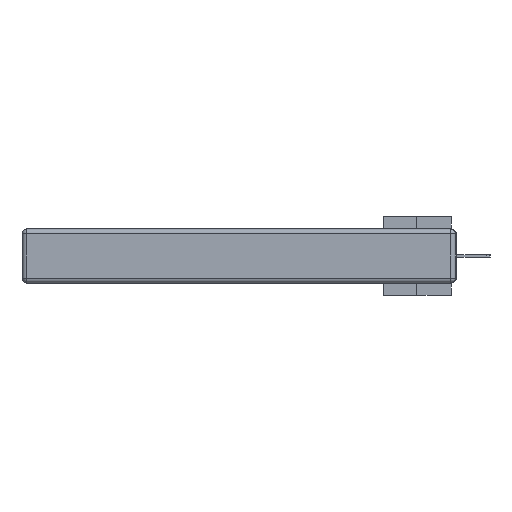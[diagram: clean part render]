
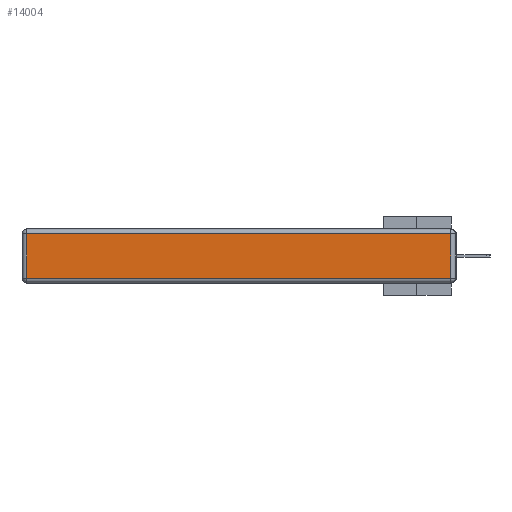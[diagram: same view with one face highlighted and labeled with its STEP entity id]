
A CAD part, left-side view. The second image highlights one B-rep face of the part: STEP entity #14004.
In plain terms, the highlighted planar face has unit normal (-1, 0, 0).
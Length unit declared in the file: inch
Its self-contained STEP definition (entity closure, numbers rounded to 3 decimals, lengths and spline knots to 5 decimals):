
#1077 = LINE ( 'NONE', #28165, #17261 ) ;
#1155 = ORIENTED_EDGE ( 'NONE', *, *, #31977, .T. ) ;
#1586 = CARTESIAN_POINT ( 'NONE',  ( 0., 0., -0.343 ) ) ;
#5888 = CARTESIAN_POINT ( 'NONE',  ( 0., 2.72, -0.313 ) ) ;
#6459 = VECTOR ( 'NONE', #10305, 39.37008 ) ;
#8306 = LINE ( 'NONE', #8474, #25198 ) ;
#8474 = CARTESIAN_POINT ( 'NONE',  ( 0., 2.75, -0.03 ) ) ;
#10305 = DIRECTION ( 'NONE',  ( 0., 0., 1. ) ) ;
#11385 = DIRECTION ( 'NONE',  ( 0., 0., 1. ) ) ;
#11484 = VERTEX_POINT ( 'NONE', #13816 ) ;
#11611 = ORIENTED_EDGE ( 'NONE', *, *, #34288, .T. ) ;
#12197 = ORIENTED_EDGE ( 'NONE', *, *, #32221, .T. ) ;
#12348 = VERTEX_POINT ( 'NONE', #5888 ) ;
#13642 = ORIENTED_EDGE ( 'NONE', *, *, #35615, .T. ) ;
#13816 = CARTESIAN_POINT ( 'NONE',  ( 0., 2.72, -0.03 ) ) ;
#14004 = ADVANCED_FACE ( 'NONE', ( #25659 ), #27163, .T. ) ;
#17261 = VECTOR ( 'NONE', #18676, 39.37008 ) ;
#18676 = DIRECTION ( 'NONE',  ( 0., 0., -1. ) ) ;
#19859 = CARTESIAN_POINT ( 'NONE',  ( 0., 0.03, -0.313 ) ) ;
#21738 = CARTESIAN_POINT ( 'NONE',  ( 0., 0., -0.313 ) ) ;
#22955 = CARTESIAN_POINT ( 'NONE',  ( 0., 0.03, -0.343 ) ) ;
#23295 = VERTEX_POINT ( 'NONE', #26764 ) ;
#25198 = VECTOR ( 'NONE', #30561, 39.37008 ) ;
#25659 = FACE_OUTER_BOUND ( 'NONE', #38600, .T. ) ;
#26764 = CARTESIAN_POINT ( 'NONE',  ( 0., 0.03, -0.03 ) ) ;
#26882 = LINE ( 'NONE', #21738, #40477 ) ;
#27163 = PLANE ( 'NONE',  #37462 ) ;
#28165 = CARTESIAN_POINT ( 'NONE',  ( 0., 2.72, -0.343 ) ) ;
#30292 = DIRECTION ( 'NONE',  ( -1., 0., 0. ) ) ;
#30561 = DIRECTION ( 'NONE',  ( 0., 1., 0. ) ) ;
#31977 = EDGE_CURVE ( 'NONE', #12348, #32867, #26882, .T. ) ;
#32221 = EDGE_CURVE ( 'NONE', #32867, #23295, #39981, .T. ) ;
#32867 = VERTEX_POINT ( 'NONE', #19859 ) ;
#34288 = EDGE_CURVE ( 'NONE', #23295, #11484, #8306, .T. ) ;
#35615 = EDGE_CURVE ( 'NONE', #11484, #12348, #1077, .T. ) ;
#37462 = AXIS2_PLACEMENT_3D ( 'NONE', #1586, #30292, #11385 ) ;
#38600 = EDGE_LOOP ( 'NONE', ( #1155, #12197, #11611, #13642 ) ) ;
#39981 = LINE ( 'NONE', #22955, #6459 ) ;
#40395 = DIRECTION ( 'NONE',  ( 0., -1., 0. ) ) ;
#40477 = VECTOR ( 'NONE', #40395, 39.37008 ) ;
